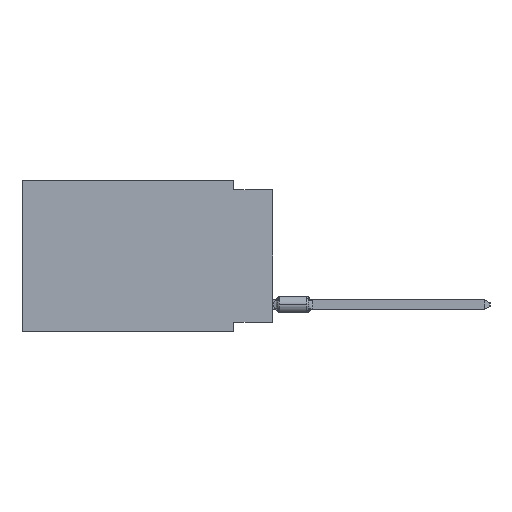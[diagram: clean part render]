
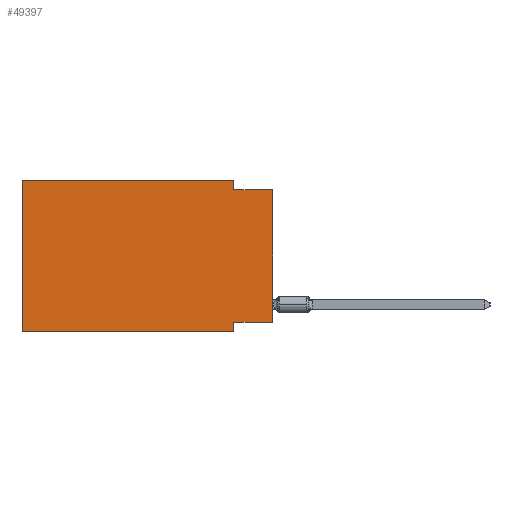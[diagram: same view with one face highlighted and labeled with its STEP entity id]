
A CAD part, left-side view. The second image highlights one B-rep face of the part: STEP entity #49397.
In plain terms, the highlighted planar face has unit normal (-1, 0, 0).
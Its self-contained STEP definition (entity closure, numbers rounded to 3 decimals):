
#308 = DIRECTION ( 'NONE',  ( 0., 0., 1. ) ) ;
#439 = DIRECTION ( 'NONE',  ( 0., 0., -1. ) ) ;
#1149 = VECTOR ( 'NONE', #7496, 1000. ) ;
#3373 = CARTESIAN_POINT ( 'NONE',  ( 0., 2.54, 0. ) ) ;
#3932 = VERTEX_POINT ( 'NONE', #3373 ) ;
#4219 = CARTESIAN_POINT ( 'NONE',  ( 0., 2.54, -9.906 ) ) ;
#7102 = VERTEX_POINT ( 'NONE', #4219 ) ;
#7496 = DIRECTION ( 'NONE',  ( 0., -1., 0. ) ) ;
#8344 = VERTEX_POINT ( 'NONE', #39279 ) ;
#8663 = DIRECTION ( 'NONE',  ( 1., 0., 0. ) ) ;
#11601 = EDGE_LOOP ( 'NONE', ( #30733, #46230, #24653, #37439, #12380, #24485, #13841, #31702 ) ) ;
#12380 = ORIENTED_EDGE ( 'NONE', *, *, #24691, .F. ) ;
#13841 = ORIENTED_EDGE ( 'NONE', *, *, #36868, .F. ) ;
#13851 = CARTESIAN_POINT ( 'NONE',  ( 0., 2.54, -9.906 ) ) ;
#15407 = LINE ( 'NONE', #43330, #35518 ) ;
#17013 = VECTOR ( 'NONE', #40346, 1000. ) ;
#17214 = EDGE_CURVE ( 'NONE', #33078, #26241, #38025, .T. ) ;
#18461 = EDGE_CURVE ( 'NONE', #33078, #8344, #38241, .T. ) ;
#20089 = LINE ( 'NONE', #13851, #23571 ) ;
#20878 = CARTESIAN_POINT ( 'NONE',  ( 0., 16.383, -9.906 ) ) ;
#21500 = EDGE_CURVE ( 'NONE', #46654, #3932, #54197, .T. ) ;
#23571 = VECTOR ( 'NONE', #24498, 1000. ) ;
#23937 = AXIS2_PLACEMENT_3D ( 'NONE', #42557, #8663, #439 ) ;
#24485 = ORIENTED_EDGE ( 'NONE', *, *, #29394, .T. ) ;
#24498 = DIRECTION ( 'NONE',  ( 0., 0., -1. ) ) ;
#24653 = ORIENTED_EDGE ( 'NONE', *, *, #44898, .F. ) ;
#24691 = EDGE_CURVE ( 'NONE', #31832, #46654, #15407, .T. ) ;
#26241 = VERTEX_POINT ( 'NONE', #59085 ) ;
#27364 = CARTESIAN_POINT ( 'NONE',  ( 0., 0., -9.271 ) ) ;
#27580 = CARTESIAN_POINT ( 'NONE',  ( 0., 0., -0.635 ) ) ;
#27680 = DIRECTION ( 'NONE',  ( 0., 1., 0. ) ) ;
#27947 = VECTOR ( 'NONE', #27680, 1000. ) ;
#28809 = CARTESIAN_POINT ( 'NONE',  ( 0., 0., -9.271 ) ) ;
#29394 = EDGE_CURVE ( 'NONE', #31832, #7102, #53849, .T. ) ;
#30191 = VERTEX_POINT ( 'NONE', #33281 ) ;
#30379 = CARTESIAN_POINT ( 'NONE',  ( 0., 2.54, 0. ) ) ;
#30697 = LINE ( 'NONE', #30379, #49755 ) ;
#30733 = ORIENTED_EDGE ( 'NONE', *, *, #18461, .T. ) ;
#31674 = EDGE_CURVE ( 'NONE', #30191, #8344, #41077, .T. ) ;
#31702 = ORIENTED_EDGE ( 'NONE', *, *, #17214, .F. ) ;
#31832 = VERTEX_POINT ( 'NONE', #43545 ) ;
#33078 = VERTEX_POINT ( 'NONE', #28809 ) ;
#33281 = CARTESIAN_POINT ( 'NONE',  ( 0., 2.54, -0.635 ) ) ;
#34787 = CARTESIAN_POINT ( 'NONE',  ( 0., 16.383, 0. ) ) ;
#35518 = VECTOR ( 'NONE', #308, 1000. ) ;
#36868 = EDGE_CURVE ( 'NONE', #26241, #7102, #20089, .T. ) ;
#37439 = ORIENTED_EDGE ( 'NONE', *, *, #21500, .F. ) ;
#38025 = LINE ( 'NONE', #27364, #27947 ) ;
#38241 = LINE ( 'NONE', #47665, #54090 ) ;
#39279 = CARTESIAN_POINT ( 'NONE',  ( 0., 0., -0.635 ) ) ;
#40346 = DIRECTION ( 'NONE',  ( 0., -1., 0. ) ) ;
#41077 = LINE ( 'NONE', #27580, #1149 ) ;
#42557 = CARTESIAN_POINT ( 'NONE',  ( 0., 16.383, 0. ) ) ;
#43330 = CARTESIAN_POINT ( 'NONE',  ( 0., 16.383, 0. ) ) ;
#43468 = PLANE ( 'NONE',  #23937 ) ;
#43545 = CARTESIAN_POINT ( 'NONE',  ( 0., 16.383, -9.906 ) ) ;
#44898 = EDGE_CURVE ( 'NONE', #3932, #30191, #30697, .T. ) ;
#46230 = ORIENTED_EDGE ( 'NONE', *, *, #31674, .F. ) ;
#46654 = VERTEX_POINT ( 'NONE', #55755 ) ;
#47570 = FACE_OUTER_BOUND ( 'NONE', #11601, .T. ) ;
#47665 = CARTESIAN_POINT ( 'NONE',  ( 0., 0., 0. ) ) ;
#49397 = ADVANCED_FACE ( 'NONE', ( #47570 ), #43468, .F. ) ;
#49755 = VECTOR ( 'NONE', #59562, 1000. ) ;
#53849 = LINE ( 'NONE', #20878, #17013 ) ;
#53894 = DIRECTION ( 'NONE',  ( 0., -1., 0. ) ) ;
#54090 = VECTOR ( 'NONE', #57688, 1000. ) ;
#54197 = LINE ( 'NONE', #34787, #59423 ) ;
#55755 = CARTESIAN_POINT ( 'NONE',  ( 0., 16.383, 0. ) ) ;
#57688 = DIRECTION ( 'NONE',  ( 0., 0., 1. ) ) ;
#59085 = CARTESIAN_POINT ( 'NONE',  ( 0., 2.54, -9.271 ) ) ;
#59423 = VECTOR ( 'NONE', #53894, 1000. ) ;
#59562 = DIRECTION ( 'NONE',  ( 0., 0., -1. ) ) ;
